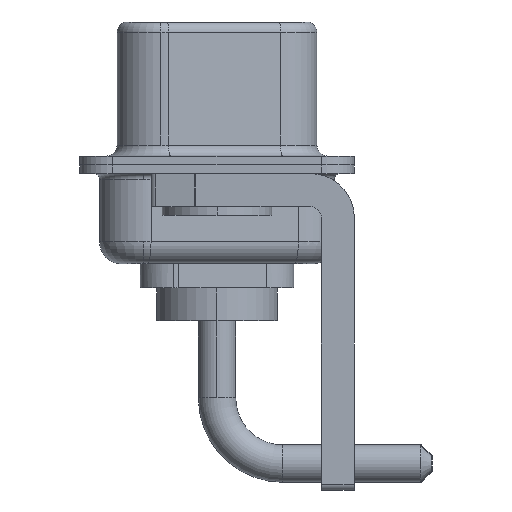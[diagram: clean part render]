
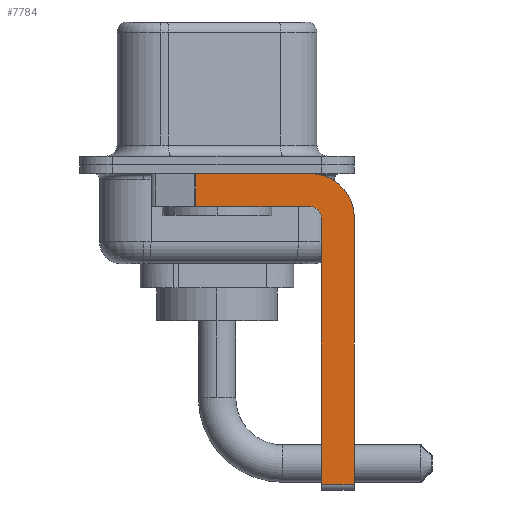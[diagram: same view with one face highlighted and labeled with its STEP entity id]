
A CAD part, left-side view. The second image highlights one B-rep face of the part: STEP entity #7784.
In plain terms, the highlighted planar face has unit normal (-1, 0, 0).
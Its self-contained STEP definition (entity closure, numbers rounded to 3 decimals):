
#129 = CARTESIAN_POINT ( 'NONE',  ( -2.9, 0.978, -0.4 ) ) ;
#419 = EDGE_CURVE ( 'NONE', #13394, #1435, #6857, .T. ) ;
#515 = EDGE_LOOP ( 'NONE', ( #12764, #9847, #1711, #12511, #723, #1861, #14228, #3090 ) ) ;
#666 = CARTESIAN_POINT ( 'NONE',  ( -2.9, 0.978, -1.9 ) ) ;
#723 = ORIENTED_EDGE ( 'NONE', *, *, #11240, .F. ) ;
#1435 = VERTEX_POINT ( 'NONE', #13606 ) ;
#1502 = CARTESIAN_POINT ( 'NONE',  ( -2.9, -4.25, -1.9 ) ) ;
#1684 = VECTOR ( 'NONE', #10185, 1000. ) ;
#1711 = ORIENTED_EDGE ( 'NONE', *, *, #12517, .F. ) ;
#1841 = EDGE_CURVE ( 'NONE', #9523, #7974, #10167, .T. ) ;
#1861 = ORIENTED_EDGE ( 'NONE', *, *, #6326, .T. ) ;
#2266 = CARTESIAN_POINT ( 'NONE',  ( -2.9, -4.75, -14.8 ) ) ;
#2346 = LINE ( 'NONE', #14269, #7683 ) ;
#2351 = DIRECTION ( 'NONE',  ( 1., 0., 0. ) ) ;
#2459 = VECTOR ( 'NONE', #9659, 1000. ) ;
#2624 = EDGE_CURVE ( 'NONE', #15003, #6381, #8808, .T. ) ;
#3090 = ORIENTED_EDGE ( 'NONE', *, *, #14170, .F. ) ;
#3166 = EDGE_CURVE ( 'NONE', #15003, #13907, #3195, .T. ) ;
#3195 = LINE ( 'NONE', #11188, #1684 ) ;
#3205 = CARTESIAN_POINT ( 'NONE',  ( -2.9, -6.25, -2.4 ) ) ;
#3968 = AXIS2_PLACEMENT_3D ( 'NONE', #12803, #2351, #6790 ) ;
#3971 = CARTESIAN_POINT ( 'NONE',  ( -2.9, -4.75, -2.4 ) ) ;
#4112 = CARTESIAN_POINT ( 'NONE',  ( -2.9, -4.25, -0.4 ) ) ;
#4246 = CARTESIAN_POINT ( 'NONE',  ( -2.9, 3., -0.4 ) ) ;
#4305 = CARTESIAN_POINT ( 'NONE',  ( -2.9, -4.25, -2.4 ) ) ;
#5165 = LINE ( 'NONE', #14420, #2459 ) ;
#5434 = DIRECTION ( 'NONE',  ( -1., 0., 0. ) ) ;
#5917 = DIRECTION ( 'NONE',  ( 0., 0., -1. ) ) ;
#6326 = EDGE_CURVE ( 'NONE', #13613, #1435, #5165, .T. ) ;
#6381 = VERTEX_POINT ( 'NONE', #4112 ) ;
#6451 = DIRECTION ( 'NONE',  ( 0., -1., 0. ) ) ;
#6635 = DIRECTION ( 'NONE',  ( 0., 0., -1. ) ) ;
#6790 = DIRECTION ( 'NONE',  ( 0., 0., -1. ) ) ;
#6857 = LINE ( 'NONE', #3205, #8861 ) ;
#7683 = VECTOR ( 'NONE', #11806, 1000. ) ;
#7784 = ADVANCED_FACE ( 'NONE', ( #13964 ), #11662, .F. ) ;
#7974 = VERTEX_POINT ( 'NONE', #1502 ) ;
#7987 = AXIS2_PLACEMENT_3D ( 'NONE', #4305, #5434, #10299 ) ;
#8156 = CARTESIAN_POINT ( 'NONE',  ( -2.9, -4.75, -14.55 ) ) ;
#8808 = LINE ( 'NONE', #4246, #10177 ) ;
#8861 = VECTOR ( 'NONE', #6635, 1000. ) ;
#9523 = VERTEX_POINT ( 'NONE', #3971 ) ;
#9659 = DIRECTION ( 'NONE',  ( 0., -1., 0. ) ) ;
#9847 = ORIENTED_EDGE ( 'NONE', *, *, #3166, .T. ) ;
#10167 = CIRCLE ( 'NONE', #7987, 0.5 ) ;
#10177 = VECTOR ( 'NONE', #6451, 1000. ) ;
#10185 = DIRECTION ( 'NONE',  ( 0., 0., -1. ) ) ;
#10299 = DIRECTION ( 'NONE',  ( 0., 0., 1. ) ) ;
#10425 = DIRECTION ( 'NONE',  ( 0., 0., 1. ) ) ;
#10827 = CARTESIAN_POINT ( 'NONE',  ( -2.9, -6.25, -2.4 ) ) ;
#11104 = AXIS2_PLACEMENT_3D ( 'NONE', #13088, #14337, #5917 ) ;
#11188 = CARTESIAN_POINT ( 'NONE',  ( -2.9, 0.978, -1.9 ) ) ;
#11240 = EDGE_CURVE ( 'NONE', #13613, #9523, #12720, .T. ) ;
#11662 = PLANE ( 'NONE',  #3968 ) ;
#11806 = DIRECTION ( 'NONE',  ( 0., 1., 0. ) ) ;
#12511 = ORIENTED_EDGE ( 'NONE', *, *, #1841, .F. ) ;
#12517 = EDGE_CURVE ( 'NONE', #7974, #13907, #2346, .T. ) ;
#12551 = VECTOR ( 'NONE', #10425, 1000. ) ;
#12720 = LINE ( 'NONE', #2266, #12551 ) ;
#12764 = ORIENTED_EDGE ( 'NONE', *, *, #2624, .F. ) ;
#12803 = CARTESIAN_POINT ( 'NONE',  ( -2.9, -4.25, -2.4 ) ) ;
#13088 = CARTESIAN_POINT ( 'NONE',  ( -2.9, -4.25, -2.4 ) ) ;
#13394 = VERTEX_POINT ( 'NONE', #10827 ) ;
#13606 = CARTESIAN_POINT ( 'NONE',  ( -2.9, -6.25, -14.55 ) ) ;
#13613 = VERTEX_POINT ( 'NONE', #8156 ) ;
#13907 = VERTEX_POINT ( 'NONE', #666 ) ;
#13964 = FACE_OUTER_BOUND ( 'NONE', #515, .T. ) ;
#14170 = EDGE_CURVE ( 'NONE', #6381, #13394, #14810, .T. ) ;
#14228 = ORIENTED_EDGE ( 'NONE', *, *, #419, .F. ) ;
#14269 = CARTESIAN_POINT ( 'NONE',  ( -2.9, -4.25, -1.9 ) ) ;
#14337 = DIRECTION ( 'NONE',  ( 1., 0., 0. ) ) ;
#14420 = CARTESIAN_POINT ( 'NONE',  ( -2.9, -4.25, -14.55 ) ) ;
#14810 = CIRCLE ( 'NONE', #11104, 2. ) ;
#15003 = VERTEX_POINT ( 'NONE', #129 ) ;
